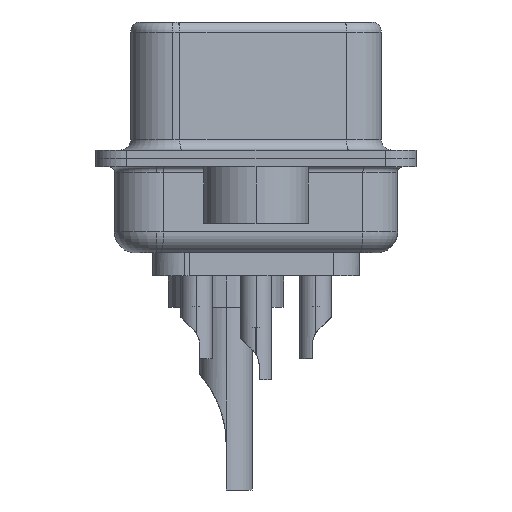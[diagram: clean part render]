
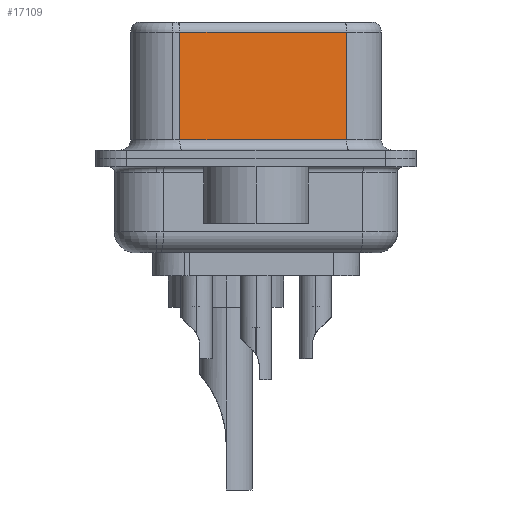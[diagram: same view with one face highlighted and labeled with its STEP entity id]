
A CAD part, left-side view. The second image highlights one B-rep face of the part: STEP entity #17109.
In plain terms, the highlighted planar face has unit normal (-0.985, -0.174, 0).
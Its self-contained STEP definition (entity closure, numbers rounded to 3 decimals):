
#1297 = VECTOR ( 'NONE', #7918, 1000. ) ;
#3076 = VECTOR ( 'NONE', #17654, 1000. ) ;
#3252 = EDGE_CURVE ( 'NONE', #24638, #7506, #9310, .T. ) ;
#5049 = FACE_OUTER_BOUND ( 'NONE', #19707, .T. ) ;
#6521 = LINE ( 'NONE', #28727, #22883 ) ;
#7506 = VERTEX_POINT ( 'NONE', #25202 ) ;
#7918 = DIRECTION ( 'NONE',  ( 0.174, -0.985, 0. ) ) ;
#8062 = EDGE_CURVE ( 'NONE', #7506, #9780, #14087, .T. ) ;
#8522 = ORIENTED_EDGE ( 'NONE', *, *, #16437, .F. ) ;
#9310 = LINE ( 'NONE', #10901, #3076 ) ;
#9780 = VERTEX_POINT ( 'NONE', #11951 ) ;
#10207 = CARTESIAN_POINT ( 'NONE',  ( 3.73, 3.628, 6.02 ) ) ;
#10901 = CARTESIAN_POINT ( 'NONE',  ( 3.73, 3.628, 6.52 ) ) ;
#11353 = ORIENTED_EDGE ( 'NONE', *, *, #3252, .T. ) ;
#11951 = CARTESIAN_POINT ( 'NONE',  ( 5.132, -4.322, 0.9 ) ) ;
#12794 = CARTESIAN_POINT ( 'NONE',  ( 5.132, -4.322, 0.9 ) ) ;
#14087 = LINE ( 'NONE', #12794, #1297 ) ;
#15158 = DIRECTION ( 'NONE',  ( -0.174, 0.985, 0. ) ) ;
#15597 = VECTOR ( 'NONE', #26865, 1000. ) ;
#16437 = EDGE_CURVE ( 'NONE', #24979, #9780, #6521, .T. ) ;
#17106 = AXIS2_PLACEMENT_3D ( 'NONE', #22456, #20033, #15158 ) ;
#17109 = ADVANCED_FACE ( 'NONE', ( #5049 ), #29091, .F. ) ;
#17654 = DIRECTION ( 'NONE',  ( 0., 0., -1. ) ) ;
#19370 = DIRECTION ( 'NONE',  ( 0., 0., -1. ) ) ;
#19707 = EDGE_LOOP ( 'NONE', ( #8522, #21393, #11353, #26525 ) ) ;
#20033 = DIRECTION ( 'NONE',  ( 0.985, 0.174, 0. ) ) ;
#21393 = ORIENTED_EDGE ( 'NONE', *, *, #25985, .T. ) ;
#22456 = CARTESIAN_POINT ( 'NONE',  ( 5.132, -4.322, 6.52 ) ) ;
#22883 = VECTOR ( 'NONE', #19370, 1000. ) ;
#24638 = VERTEX_POINT ( 'NONE', #10207 ) ;
#24979 = VERTEX_POINT ( 'NONE', #27227 ) ;
#25062 = LINE ( 'NONE', #26669, #15597 ) ;
#25202 = CARTESIAN_POINT ( 'NONE',  ( 3.73, 3.628, 0.9 ) ) ;
#25985 = EDGE_CURVE ( 'NONE', #24979, #24638, #25062, .T. ) ;
#26525 = ORIENTED_EDGE ( 'NONE', *, *, #8062, .T. ) ;
#26669 = CARTESIAN_POINT ( 'NONE',  ( 5.132, -4.322, 6.02 ) ) ;
#26865 = DIRECTION ( 'NONE',  ( -0.174, 0.985, 0. ) ) ;
#27227 = CARTESIAN_POINT ( 'NONE',  ( 5.132, -4.322, 6.02 ) ) ;
#28727 = CARTESIAN_POINT ( 'NONE',  ( 5.132, -4.322, 6.52 ) ) ;
#29091 = PLANE ( 'NONE',  #17106 ) ;
